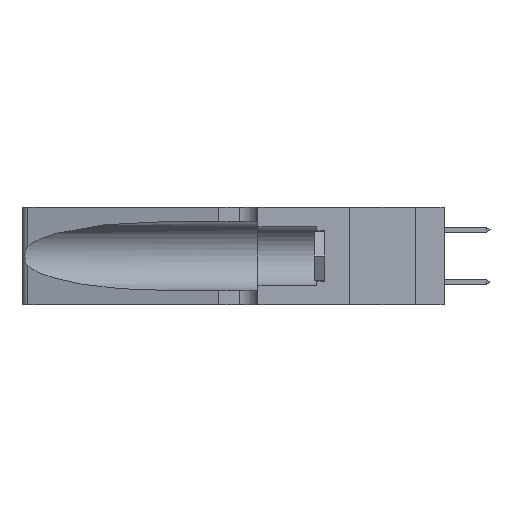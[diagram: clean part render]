
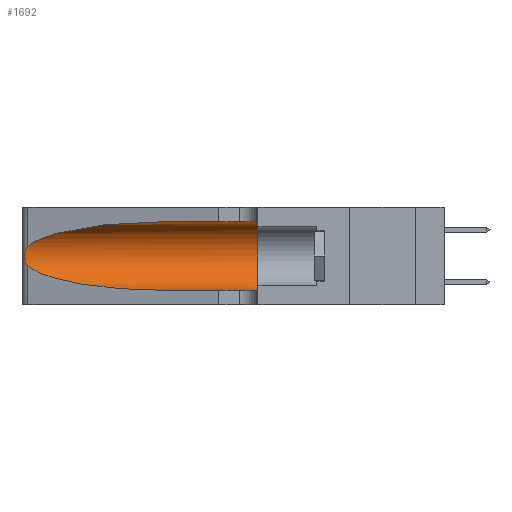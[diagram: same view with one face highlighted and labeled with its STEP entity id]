
A CAD part, left-side view. The second image highlights one B-rep face of the part: STEP entity #1692.
In plain terms, the highlighted cylindrical face has radius 3.308 mm (diameter 6.617 mm), a partial arc.
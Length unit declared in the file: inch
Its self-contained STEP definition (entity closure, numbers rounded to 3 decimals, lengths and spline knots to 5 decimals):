
#56 = EDGE_CURVE ( 'NONE', #6000, #21481, #9755, .T. ) ;
#238 = EDGE_CURVE ( 'NONE', #9931, #13674, #11787, .T. ) ;
#475 = DIRECTION ( 'NONE',  ( 0., 1., 0. ) ) ;
#687 = CARTESIAN_POINT ( 'NONE',  ( 0.26075, 1.23896, 0.178 ) ) ;
#845 = CARTESIAN_POINT ( 'NONE',  ( 0.25639, 1.23186, 0.15144 ) ) ;
#980 = CARTESIAN_POINT ( 'NONE',  ( 0.2373, 1.15595, 0.28018 ) ) ;
#1692 = ADVANCED_FACE ( 'NONE', ( #22266 ), #21751, .F. ) ;
#1707 = VERTEX_POINT ( 'NONE', #9678 ) ;
#1856 = ORIENTED_EDGE ( 'NONE', *, *, #18795, .F. ) ;
#2026 = VERTEX_POINT ( 'NONE', #3598 ) ;
#2214 = DIRECTION ( 'NONE',  ( 0., 0., 1. ) ) ;
#2504 = CARTESIAN_POINT ( 'NONE',  ( 0.25487, 1.22718, 0.22369 ) ) ;
#2634 = CARTESIAN_POINT ( 'NONE',  ( 0.1305, 0.72297, 0.31525 ) ) ;
#2936 = CARTESIAN_POINT ( 'NONE',  ( 0.25487, 1.22718, 0.14631 ) ) ;
#3397 = ORIENTED_EDGE ( 'NONE', *, *, #238, .T. ) ;
#3598 = CARTESIAN_POINT ( 'NONE',  ( 0.1305, 0.35, 0.31525 ) ) ;
#4919 = ORIENTED_EDGE ( 'NONE', *, *, #56, .T. ) ;
#5246 = DIRECTION ( 'NONE',  ( 0., -1., 0. ) ) ;
#5924 = CARTESIAN_POINT ( 'NONE',  ( 0.25487, 1.22718, 0.14631 ) ) ;
#6000 = VERTEX_POINT ( 'NONE', #6053 ) ;
#6053 = CARTESIAN_POINT ( 'NONE',  ( 0.1305, 0.72297, 0.31525 ) ) ;
#6069 = CARTESIAN_POINT ( 'NONE',  ( 0.25487, 1.22718, 0.14631 ) ) ;
#6145 = CARTESIAN_POINT ( 'NONE',  ( 0.25854, 1.2359, 0.20912 ) ) ;
#6578 = EDGE_CURVE ( 'NONE', #21481, #9931, #13201, .T. ) ;
#6616 = CARTESIAN_POINT ( 'NONE',  ( 0.1305, 0.72297, 0.05475 ) ) ;
#7015 = EDGE_LOOP ( 'NONE', ( #4919, #16381, #3397, #15361, #1856, #15077 ) ) ;
#7738 = CARTESIAN_POINT ( 'NONE',  ( 0.25555, 1.22994, 0.2215 ) ) ;
#7786 = CARTESIAN_POINT ( 'NONE',  ( 0.1305, 1.61858, 0.185 ) ) ;
#8012 = EDGE_CURVE ( 'NONE', #6000, #2026, #13441, .T. ) ;
#8152 = CARTESIAN_POINT ( 'NONE',  ( 0.18966, 0.96281, 0.05475 ) ) ;
#9114 = VECTOR ( 'NONE', #19368, 39.37008 ) ;
#9556 = CARTESIAN_POINT ( 'NONE',  ( 0.25555, 1.22993, 0.14849 ) ) ;
#9678 = CARTESIAN_POINT ( 'NONE',  ( 0.1305, 0.35, 0.05475 ) ) ;
#9755 =( BOUNDED_CURVE ( )  B_SPLINE_CURVE ( 3, ( #2634, #16552, #980, #18028 ),
 .UNSPECIFIED., .F., .F. ) 
 B_SPLINE_CURVE_WITH_KNOTS ( ( 4, 4 ),
 ( 1.5708, 2.84003 ),
 .UNSPECIFIED. ) 
 CURVE ( )  GEOMETRIC_REPRESENTATION_ITEM ( )  RATIONAL_B_SPLINE_CURVE ( ( 1., 0.87, 0.87, 1. ) ) 
 REPRESENTATION_ITEM ( '' )  );
#9931 = VERTEX_POINT ( 'NONE', #6069 ) ;
#10705 = CARTESIAN_POINT ( 'NONE',  ( 0.1305, 1.61858, 0.31525 ) ) ;
#11193 = CARTESIAN_POINT ( 'NONE',  ( 0.26017, 1.23833, 0.17102 ) ) ;
#11274 = CARTESIAN_POINT ( 'NONE',  ( 0.25856, 1.23593, 0.16098 ) ) ;
#11787 =( BOUNDED_CURVE ( )  B_SPLINE_CURVE ( 3, ( #2936, #18471, #8152, #6616 ),
 .UNSPECIFIED., .F., .F. ) 
 B_SPLINE_CURVE_WITH_KNOTS ( ( 4, 4 ),
 ( 3.44316, 4.71239 ),
 .UNSPECIFIED. ) 
 CURVE ( )  GEOMETRIC_REPRESENTATION_ITEM ( )  RATIONAL_B_SPLINE_CURVE ( ( 1., 0.87, 0.87, 1. ) ) 
 REPRESENTATION_ITEM ( '' )  );
#12254 = CARTESIAN_POINT ( 'NONE',  ( 0.1305, 0.35, 0.185 ) ) ;
#12387 = CARTESIAN_POINT ( 'NONE',  ( 0.1305, 1.61858, 0.05475 ) ) ;
#13201 = B_SPLINE_CURVE_WITH_KNOTS ( 'NONE', 3,
 ( #2504, #7738, #19930, #16428, #6145, #21530, #21371, #687, #11193, #11274, #14536, #845, #9556, #5924 ),
 .UNSPECIFIED., .F., .F.,
 ( 4, 2, 2, 2, 2, 2, 4 ),
 ( 0., 0.00027, 0.00053, 0.00107, 0.0016, 0.00187, 0.00214 ),
 .UNSPECIFIED. ) ;
#13441 = LINE ( 'NONE', #10705, #9114 ) ;
#13674 = VERTEX_POINT ( 'NONE', #17661 ) ;
#14141 = EDGE_CURVE ( 'NONE', #13674, #1707, #20114, .T. ) ;
#14536 = CARTESIAN_POINT ( 'NONE',  ( 0.25789, 1.23486, 0.15765 ) ) ;
#15077 = ORIENTED_EDGE ( 'NONE', *, *, #8012, .F. ) ;
#15361 = ORIENTED_EDGE ( 'NONE', *, *, #14141, .T. ) ;
#16381 = ORIENTED_EDGE ( 'NONE', *, *, #6578, .T. ) ;
#16428 = CARTESIAN_POINT ( 'NONE',  ( 0.25787, 1.23484, 0.2124 ) ) ;
#16552 = CARTESIAN_POINT ( 'NONE',  ( 0.18966, 0.96281, 0.31525 ) ) ;
#17661 = CARTESIAN_POINT ( 'NONE',  ( 0.1305, 0.72297, 0.05475 ) ) ;
#17689 = CARTESIAN_POINT ( 'NONE',  ( 0.25487, 1.22718, 0.22369 ) ) ;
#18028 = CARTESIAN_POINT ( 'NONE',  ( 0.25487, 1.22718, 0.22369 ) ) ;
#18471 = CARTESIAN_POINT ( 'NONE',  ( 0.2373, 1.15595, 0.08982 ) ) ;
#18795 = EDGE_CURVE ( 'NONE', #2026, #1707, #21336, .T. ) ;
#19368 = DIRECTION ( 'NONE',  ( 0., -1., 0. ) ) ;
#19592 = VECTOR ( 'NONE', #5246, 39.37008 ) ;
#19930 = CARTESIAN_POINT ( 'NONE',  ( 0.25639, 1.23184, 0.21858 ) ) ;
#20114 = LINE ( 'NONE', #12387, #19592 ) ;
#21336 = CIRCLE ( 'NONE', #21873, 0.13025 ) ;
#21371 = CARTESIAN_POINT ( 'NONE',  ( 0.26075, 1.23896, 0.19203 ) ) ;
#21481 = VERTEX_POINT ( 'NONE', #17689 ) ;
#21530 = CARTESIAN_POINT ( 'NONE',  ( 0.26018, 1.23835, 0.19895 ) ) ;
#21576 = DIRECTION ( 'NONE',  ( 0., -1., 0. ) ) ;
#21658 = DIRECTION ( 'NONE',  ( 0., 0., -1. ) ) ;
#21751 = CYLINDRICAL_SURFACE ( 'NONE', #21907, 0.13025 ) ;
#21873 = AXIS2_PLACEMENT_3D ( 'NONE', #12254, #475, #2214 ) ;
#21907 = AXIS2_PLACEMENT_3D ( 'NONE', #7786, #21576, #21658 ) ;
#22266 = FACE_OUTER_BOUND ( 'NONE', #7015, .T. ) ;
